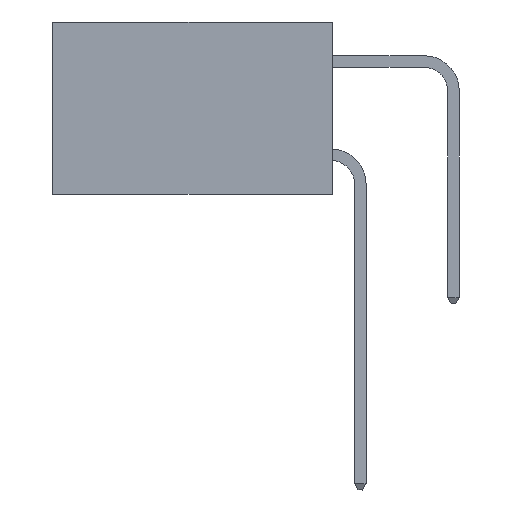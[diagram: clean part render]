
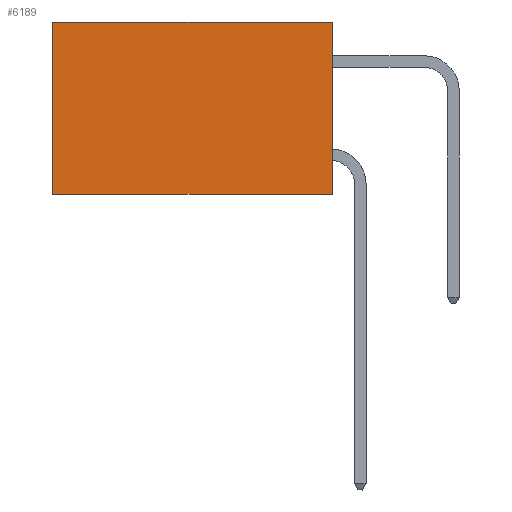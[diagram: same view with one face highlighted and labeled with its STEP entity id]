
A CAD part, left-side view. The second image highlights one B-rep face of the part: STEP entity #6189.
In plain terms, the highlighted planar face has unit normal (-1, 0, 0).
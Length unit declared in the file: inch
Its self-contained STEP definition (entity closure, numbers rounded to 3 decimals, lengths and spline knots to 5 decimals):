
#1333 = VECTOR ( 'NONE', #20272, 39.37008 ) ;
#1373 = DIRECTION ( 'NONE',  ( 1., 0., 0. ) ) ;
#1694 = CARTESIAN_POINT ( 'NONE',  ( 0.298, 0.6, -0.37 ) ) ;
#3109 = VERTEX_POINT ( 'NONE', #12929 ) ;
#3313 = CARTESIAN_POINT ( 'NONE',  ( 0.298, 0.6, 0. ) ) ;
#4287 = ORIENTED_EDGE ( 'NONE', *, *, #17641, .T. ) ;
#4347 = VERTEX_POINT ( 'NONE', #19025 ) ;
#4613 = DIRECTION ( 'NONE',  ( 0., 0., -1. ) ) ;
#5028 = VECTOR ( 'NONE', #16323, 39.37008 ) ;
#6189 = ADVANCED_FACE ( 'NONE', ( #6974 ), #7795, .F. ) ;
#6974 = FACE_OUTER_BOUND ( 'NONE', #18693, .T. ) ;
#7630 = ORIENTED_EDGE ( 'NONE', *, *, #9404, .F. ) ;
#7795 = PLANE ( 'NONE',  #11958 ) ;
#8210 = CARTESIAN_POINT ( 'NONE',  ( 0.298, 0., -0.37 ) ) ;
#9206 = VECTOR ( 'NONE', #4613, 39.37008 ) ;
#9404 = EDGE_CURVE ( 'NONE', #16222, #4347, #17679, .T. ) ;
#10305 = ORIENTED_EDGE ( 'NONE', *, *, #11825, .T. ) ;
#11738 = LINE ( 'NONE', #3313, #9206 ) ;
#11825 = EDGE_CURVE ( 'NONE', #16222, #3109, #13471, .T. ) ;
#11958 = AXIS2_PLACEMENT_3D ( 'NONE', #20349, #1373, #17385 ) ;
#12451 = LINE ( 'NONE', #8210, #5028 ) ;
#12870 = CARTESIAN_POINT ( 'NONE',  ( 0.298, 0., 0. ) ) ;
#12929 = CARTESIAN_POINT ( 'NONE',  ( 0.298, 0.6, 0. ) ) ;
#13471 = LINE ( 'NONE', #13899, #1333 ) ;
#13899 = CARTESIAN_POINT ( 'NONE',  ( 0.298, 0., 0. ) ) ;
#14986 = ORIENTED_EDGE ( 'NONE', *, *, #17701, .F. ) ;
#15536 = DIRECTION ( 'NONE',  ( 0., 0., -1. ) ) ;
#16222 = VERTEX_POINT ( 'NONE', #12870 ) ;
#16323 = DIRECTION ( 'NONE',  ( 0., 1., 0. ) ) ;
#16562 = VERTEX_POINT ( 'NONE', #1694 ) ;
#17385 = DIRECTION ( 'NONE',  ( 0., 0., -1. ) ) ;
#17641 = EDGE_CURVE ( 'NONE', #3109, #16562, #11738, .T. ) ;
#17679 = LINE ( 'NONE', #20185, #19905 ) ;
#17701 = EDGE_CURVE ( 'NONE', #4347, #16562, #12451, .T. ) ;
#18693 = EDGE_LOOP ( 'NONE', ( #4287, #14986, #7630, #10305 ) ) ;
#19025 = CARTESIAN_POINT ( 'NONE',  ( 0.298, 0., -0.37 ) ) ;
#19905 = VECTOR ( 'NONE', #15536, 39.37008 ) ;
#20185 = CARTESIAN_POINT ( 'NONE',  ( 0.298, 0., 0. ) ) ;
#20272 = DIRECTION ( 'NONE',  ( 0., 1., 0. ) ) ;
#20349 = CARTESIAN_POINT ( 'NONE',  ( 0.298, 0., 0. ) ) ;
